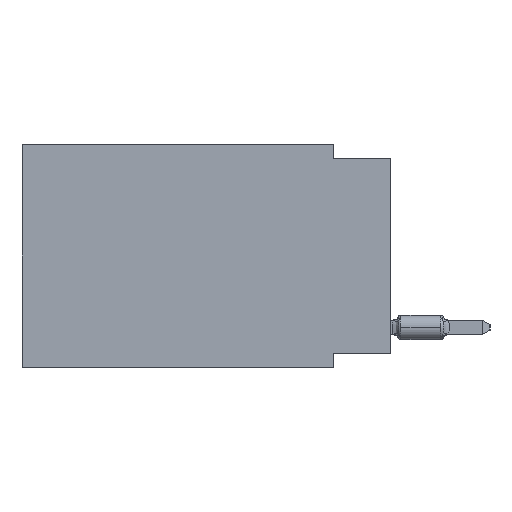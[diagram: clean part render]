
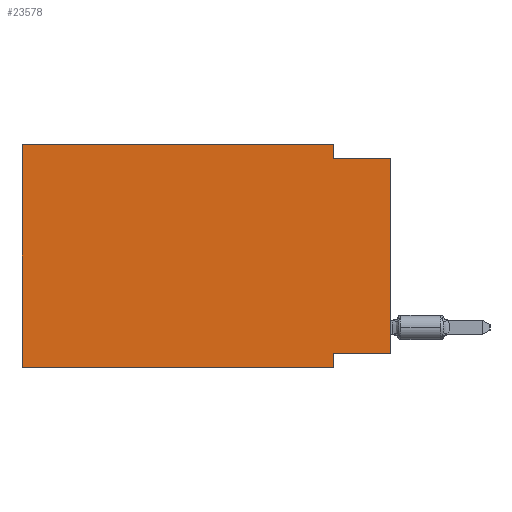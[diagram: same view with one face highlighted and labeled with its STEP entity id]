
A CAD part, left-side view. The second image highlights one B-rep face of the part: STEP entity #23578.
In plain terms, the highlighted planar face has unit normal (-1, 0, 0).
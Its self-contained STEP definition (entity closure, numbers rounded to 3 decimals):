
#236 = FACE_OUTER_BOUND ( 'NONE', #6351, .T. ) ;
#387 = LINE ( 'NONE', #5399, #12322 ) ;
#655 = CARTESIAN_POINT ( 'NONE',  ( 0., 2.54, -9.271 ) ) ;
#945 = CARTESIAN_POINT ( 'NONE',  ( 0., 2.54, -9.906 ) ) ;
#1358 = VECTOR ( 'NONE', #13165, 1000. ) ;
#1469 = EDGE_CURVE ( 'NONE', #3623, #5720, #16185, .T. ) ;
#1858 = ORIENTED_EDGE ( 'NONE', *, *, #1469, .F. ) ;
#2103 = VECTOR ( 'NONE', #21999, 1000. ) ;
#2158 = EDGE_CURVE ( 'NONE', #26489, #23585, #15120, .T. ) ;
#3462 = ORIENTED_EDGE ( 'NONE', *, *, #2158, .F. ) ;
#3623 = VERTEX_POINT ( 'NONE', #11460 ) ;
#3869 = VERTEX_POINT ( 'NONE', #25802 ) ;
#4177 = VERTEX_POINT ( 'NONE', #7725 ) ;
#4522 = AXIS2_PLACEMENT_3D ( 'NONE', #17407, #11218, #26019 ) ;
#5399 = CARTESIAN_POINT ( 'NONE',  ( 0., 16.383, -9.906 ) ) ;
#5572 = LINE ( 'NONE', #945, #11000 ) ;
#5720 = VERTEX_POINT ( 'NONE', #22530 ) ;
#5909 = CARTESIAN_POINT ( 'NONE',  ( 0., 0., 0. ) ) ;
#6125 = ORIENTED_EDGE ( 'NONE', *, *, #22779, .F. ) ;
#6351 = EDGE_LOOP ( 'NONE', ( #13033, #6125, #11119, #1858, #19721, #26565, #19309, #3462 ) ) ;
#7725 = CARTESIAN_POINT ( 'NONE',  ( 0., 2.54, -9.906 ) ) ;
#8062 = EDGE_CURVE ( 'NONE', #21338, #4177, #387, .T. ) ;
#8419 = CARTESIAN_POINT ( 'NONE',  ( 0., 16.383, 0. ) ) ;
#8799 = PLANE ( 'NONE',  #4522 ) ;
#9031 = LINE ( 'NONE', #15009, #1358 ) ;
#9166 = VECTOR ( 'NONE', #21650, 1000. ) ;
#9671 = DIRECTION ( 'NONE',  ( 0., -1., 0. ) ) ;
#11000 = VECTOR ( 'NONE', #18265, 1000. ) ;
#11119 = ORIENTED_EDGE ( 'NONE', *, *, #16858, .F. ) ;
#11218 = DIRECTION ( 'NONE',  ( 1., 0., 0. ) ) ;
#11363 = LINE ( 'NONE', #17968, #9166 ) ;
#11460 = CARTESIAN_POINT ( 'NONE',  ( 0., 16.383, 0. ) ) ;
#11532 = VECTOR ( 'NONE', #9671, 1000. ) ;
#11536 = CARTESIAN_POINT ( 'NONE',  ( 0., 16.383, 0. ) ) ;
#12322 = VECTOR ( 'NONE', #13884, 1000. ) ;
#13033 = ORIENTED_EDGE ( 'NONE', *, *, #20001, .T. ) ;
#13165 = DIRECTION ( 'NONE',  ( 0., -1., 0. ) ) ;
#13535 = VECTOR ( 'NONE', #17030, 1000. ) ;
#13884 = DIRECTION ( 'NONE',  ( 0., -1., 0. ) ) ;
#15009 = CARTESIAN_POINT ( 'NONE',  ( 0., 0., -0.635 ) ) ;
#15120 = LINE ( 'NONE', #17475, #2103 ) ;
#16185 = LINE ( 'NONE', #11536, #11532 ) ;
#16858 = EDGE_CURVE ( 'NONE', #5720, #19988, #11363, .T. ) ;
#17030 = DIRECTION ( 'NONE',  ( 0., 0., 1. ) ) ;
#17407 = CARTESIAN_POINT ( 'NONE',  ( 0., 16.383, 0. ) ) ;
#17475 = CARTESIAN_POINT ( 'NONE',  ( 0., 0., -9.271 ) ) ;
#17968 = CARTESIAN_POINT ( 'NONE',  ( 0., 2.54, 0. ) ) ;
#18023 = CARTESIAN_POINT ( 'NONE',  ( 0., 16.383, -9.906 ) ) ;
#18265 = DIRECTION ( 'NONE',  ( 0., 0., -1. ) ) ;
#19309 = ORIENTED_EDGE ( 'NONE', *, *, #27507, .F. ) ;
#19721 = ORIENTED_EDGE ( 'NONE', *, *, #23148, .F. ) ;
#19988 = VERTEX_POINT ( 'NONE', #25244 ) ;
#20001 = EDGE_CURVE ( 'NONE', #26489, #3869, #27094, .T. ) ;
#21338 = VERTEX_POINT ( 'NONE', #18023 ) ;
#21462 = CARTESIAN_POINT ( 'NONE',  ( 0., 0., -9.271 ) ) ;
#21650 = DIRECTION ( 'NONE',  ( 0., 0., -1. ) ) ;
#21999 = DIRECTION ( 'NONE',  ( 0., 1., 0. ) ) ;
#22530 = CARTESIAN_POINT ( 'NONE',  ( 0., 2.54, 0. ) ) ;
#22779 = EDGE_CURVE ( 'NONE', #19988, #3869, #9031, .T. ) ;
#23148 = EDGE_CURVE ( 'NONE', #21338, #3623, #25498, .T. ) ;
#23578 = ADVANCED_FACE ( 'NONE', ( #236 ), #8799, .F. ) ;
#23585 = VERTEX_POINT ( 'NONE', #655 ) ;
#24435 = VECTOR ( 'NONE', #27234, 1000. ) ;
#25244 = CARTESIAN_POINT ( 'NONE',  ( 0., 2.54, -0.635 ) ) ;
#25498 = LINE ( 'NONE', #8419, #13535 ) ;
#25802 = CARTESIAN_POINT ( 'NONE',  ( 0., 0., -0.635 ) ) ;
#26019 = DIRECTION ( 'NONE',  ( 0., 0., -1. ) ) ;
#26489 = VERTEX_POINT ( 'NONE', #21462 ) ;
#26565 = ORIENTED_EDGE ( 'NONE', *, *, #8062, .T. ) ;
#27094 = LINE ( 'NONE', #5909, #24435 ) ;
#27234 = DIRECTION ( 'NONE',  ( 0., 0., 1. ) ) ;
#27507 = EDGE_CURVE ( 'NONE', #23585, #4177, #5572, .T. ) ;
